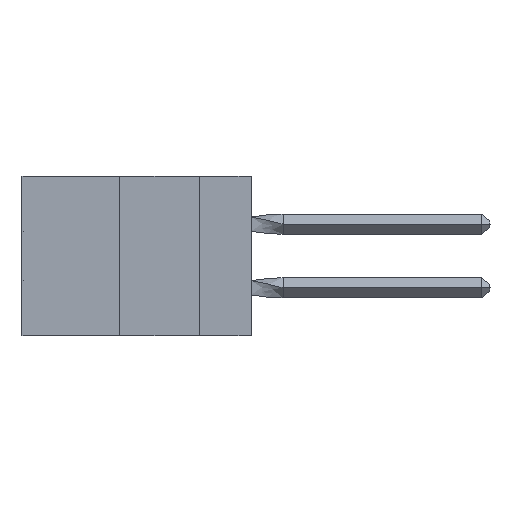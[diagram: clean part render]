
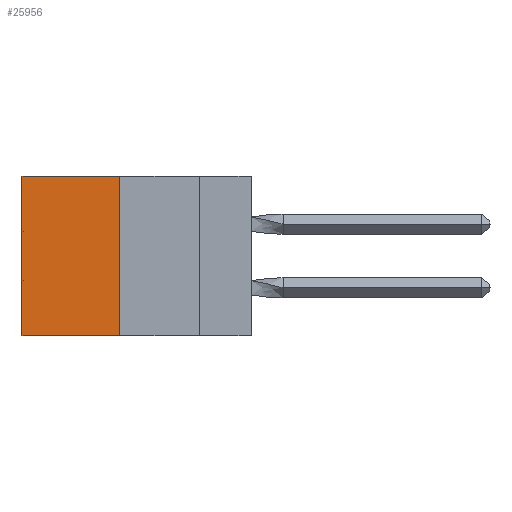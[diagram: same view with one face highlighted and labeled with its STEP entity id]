
A CAD part, left-side view. The second image highlights one B-rep face of the part: STEP entity #25956.
In plain terms, the highlighted planar face has unit normal (-1, 0, 0).
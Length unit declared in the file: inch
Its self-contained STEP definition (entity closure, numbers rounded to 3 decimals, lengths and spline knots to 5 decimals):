
#625 = VERTEX_POINT ( 'NONE', #11044 ) ;
#1025 = VECTOR ( 'NONE', #10563, 39.37008 ) ;
#1465 = FACE_OUTER_BOUND ( 'NONE', #19709, .T. ) ;
#2140 = LINE ( 'NONE', #16747, #17958 ) ;
#2830 = VECTOR ( 'NONE', #11895, 39.37008 ) ;
#4788 = ORIENTED_EDGE ( 'NONE', *, *, #6517, .F. ) ;
#6517 = EDGE_CURVE ( 'NONE', #625, #24589, #41121, .T. ) ;
#10563 = DIRECTION ( 'NONE',  ( 0., 0., -1. ) ) ;
#10708 = CARTESIAN_POINT ( 'NONE',  ( 0.305, 0.413, -0.5 ) ) ;
#11044 = CARTESIAN_POINT ( 'NONE',  ( 0.305, 0.413, -0.5 ) ) ;
#11895 = DIRECTION ( 'NONE',  ( 0., 1., 0. ) ) ;
#13092 = EDGE_CURVE ( 'NONE', #42988, #24589, #2140, .T. ) ;
#13273 = EDGE_CURVE ( 'NONE', #20916, #625, #24222, .T. ) ;
#15444 = CARTESIAN_POINT ( 'NONE',  ( 0.305, 0.413, 0. ) ) ;
#15970 = ORIENTED_EDGE ( 'NONE', *, *, #16368, .T. ) ;
#16368 = EDGE_CURVE ( 'NONE', #20916, #42988, #41245, .T. ) ;
#16747 = CARTESIAN_POINT ( 'NONE',  ( 0.305, 0.72, -0.5 ) ) ;
#17958 = VECTOR ( 'NONE', #40247, 39.37008 ) ;
#19709 = EDGE_LOOP ( 'NONE', ( #21761, #4788, #40721, #15970 ) ) ;
#20449 = CARTESIAN_POINT ( 'NONE',  ( 0.305, 0.413, -0.5 ) ) ;
#20480 = CARTESIAN_POINT ( 'NONE',  ( 0.305, 0.413, -0.5 ) ) ;
#20585 = CARTESIAN_POINT ( 'NONE',  ( 0.305, 0.72, 0. ) ) ;
#20842 = CARTESIAN_POINT ( 'NONE',  ( 0.305, 0.72, -0.5 ) ) ;
#20916 = VERTEX_POINT ( 'NONE', #15444 ) ;
#21761 = ORIENTED_EDGE ( 'NONE', *, *, #13092, .T. ) ;
#24222 = LINE ( 'NONE', #10708, #1025 ) ;
#24589 = VERTEX_POINT ( 'NONE', #20842 ) ;
#25956 = ADVANCED_FACE ( 'NONE', ( #1465 ), #37195, .F. ) ;
#31861 = AXIS2_PLACEMENT_3D ( 'NONE', #20449, #33532, #34100 ) ;
#32597 = VECTOR ( 'NONE', #38448, 39.37008 ) ;
#33532 = DIRECTION ( 'NONE',  ( 1., 0., 0. ) ) ;
#34100 = DIRECTION ( 'NONE',  ( 0., 0., -1. ) ) ;
#37195 = PLANE ( 'NONE',  #31861 ) ;
#38448 = DIRECTION ( 'NONE',  ( 0., 1., 0. ) ) ;
#38698 = CARTESIAN_POINT ( 'NONE',  ( 0.305, 0.413, 0. ) ) ;
#40247 = DIRECTION ( 'NONE',  ( 0., 0., -1. ) ) ;
#40721 = ORIENTED_EDGE ( 'NONE', *, *, #13273, .F. ) ;
#41121 = LINE ( 'NONE', #20480, #32597 ) ;
#41245 = LINE ( 'NONE', #38698, #2830 ) ;
#42988 = VERTEX_POINT ( 'NONE', #20585 ) ;
